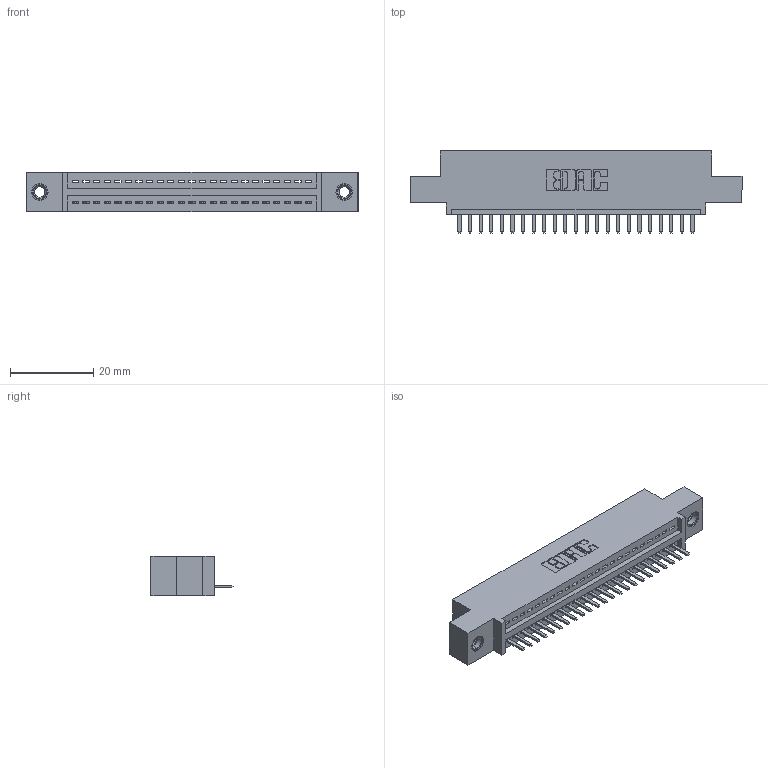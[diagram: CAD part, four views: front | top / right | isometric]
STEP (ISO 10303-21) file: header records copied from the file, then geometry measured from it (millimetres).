
FILE_DESCRIPTION (( 'STEP AP203' ), '1' );
FILE_NAME ('395-023-520-407.STEP', '2019-10-18T04:01:15', ( '' ), ( '' ), 'SwSTEP 2.0', 'SolidWorks 2016', '' );
FILE_SCHEMA (( 'CONFIG_CONTROL_DESIGN' ));
Length unit declared in the file: inch
Products named in the file (4): 345-292-001_345-293-120; 345 Part_0.110 Offset - 0.156 Dia-TI; 345-250-001_345-250-005-103; 395-023-520-407
Assembly tree (26 placements, depth 2):
  395-023-520-407
    345 Part_0.110 Offset - 0.156 Dia-TI
    345-292-001_345-293-120  x23
    345-250-001_345-250-005-103  x2
Bounding box: 79.63 x 19.68 x 9.4 mm (x, y, z)
Volume: 7254.6 mm3; surface area: 9280.4 mm2
Topology: 26 solids, 26 shells, 1616 faces, 4721 edges, 3078 vertices
Faces by surface type: plane 1082, cylinder 518, cone 12, torus 4
Entity records: 21300 total; most frequent: CARTESIAN_POINT 3684, ORIENTED_EDGE 3622, DIRECTION 3259, EDGE_CURVE 1811, VECTOR 1563, LINE 1563, VERTEX_POINT 1200, AXIS2_PLACEMENT_3D 848
